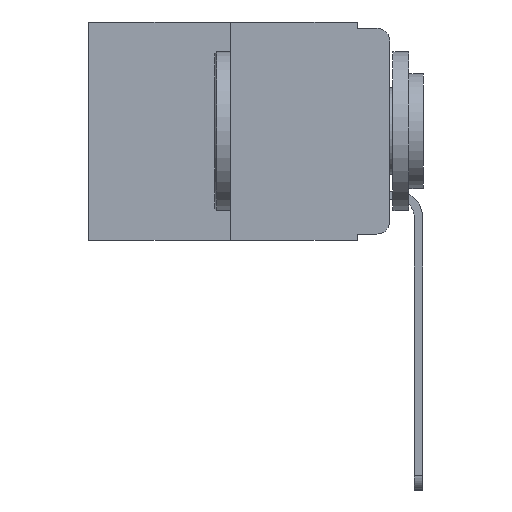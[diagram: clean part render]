
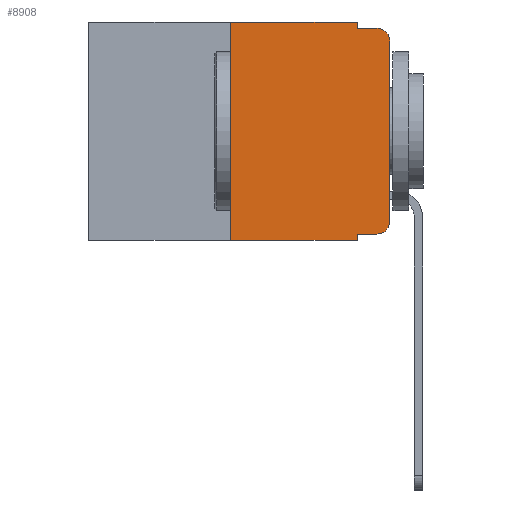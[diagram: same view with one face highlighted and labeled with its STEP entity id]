
A CAD part, left-side view. The second image highlights one B-rep face of the part: STEP entity #8908.
In plain terms, the highlighted planar face has unit normal (-1, 0, 0).
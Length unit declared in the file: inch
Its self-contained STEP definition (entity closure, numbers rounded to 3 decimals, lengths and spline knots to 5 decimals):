
#420 = CARTESIAN_POINT ( 'NONE',  ( 0., 0.473, 0. ) ) ;
#511 = CARTESIAN_POINT ( 'NONE',  ( 0., 0.051, -0.333 ) ) ;
#527 = AXIS2_PLACEMENT_3D ( 'NONE', #420, #4409, #4453 ) ;
#925 = CARTESIAN_POINT ( 'NONE',  ( 0., 0.051, -0.01 ) ) ;
#1046 = VECTOR ( 'NONE', #10687, 39.37008 ) ;
#1094 = DIRECTION ( 'NONE',  ( 0., 0., -1. ) ) ;
#1204 = LINE ( 'NONE', #7359, #10614 ) ;
#1494 = VERTEX_POINT ( 'NONE', #3408 ) ;
#1612 = CARTESIAN_POINT ( 'NONE',  ( 0., 0.02, -0.01 ) ) ;
#1719 = AXIS2_PLACEMENT_3D ( 'NONE', #12759, #5853, #1752 ) ;
#1752 = DIRECTION ( 'NONE',  ( 0., 0., -1. ) ) ;
#1886 = ORIENTED_EDGE ( 'NONE', *, *, #8521, .T. ) ;
#1899 = CARTESIAN_POINT ( 'NONE',  ( 0., 0.02, -0.03 ) ) ;
#1939 = ORIENTED_EDGE ( 'NONE', *, *, #9446, .T. ) ;
#1978 = DIRECTION ( 'NONE',  ( 0., 0., -1. ) ) ;
#2279 = CARTESIAN_POINT ( 'NONE',  ( 0., 0., 0. ) ) ;
#2830 = VERTEX_POINT ( 'NONE', #925 ) ;
#2940 = VERTEX_POINT ( 'NONE', #6816 ) ;
#2972 = EDGE_CURVE ( 'NONE', #7013, #5852, #4363, .T. ) ;
#3397 = EDGE_CURVE ( 'NONE', #2940, #4117, #1204, .T. ) ;
#3408 = CARTESIAN_POINT ( 'NONE',  ( 0., 0.25, -0.343 ) ) ;
#3981 = ORIENTED_EDGE ( 'NONE', *, *, #4809, .F. ) ;
#4117 = VERTEX_POINT ( 'NONE', #8091 ) ;
#4363 = LINE ( 'NONE', #10777, #1046 ) ;
#4409 = DIRECTION ( 'NONE',  ( 1., 0., 0. ) ) ;
#4453 = DIRECTION ( 'NONE',  ( 0., 0., -1. ) ) ;
#4462 = LINE ( 'NONE', #2279, #7758 ) ;
#4608 = VERTEX_POINT ( 'NONE', #1612 ) ;
#4751 = VERTEX_POINT ( 'NONE', #5186 ) ;
#4809 = EDGE_CURVE ( 'NONE', #4117, #2830, #5350, .T. ) ;
#4914 = EDGE_CURVE ( 'NONE', #2830, #4608, #7776, .T. ) ;
#4993 = VECTOR ( 'NONE', #1094, 39.37008 ) ;
#5142 = ORIENTED_EDGE ( 'NONE', *, *, #10206, .F. ) ;
#5186 = CARTESIAN_POINT ( 'NONE',  ( 0., 0., -0.313 ) ) ;
#5350 = LINE ( 'NONE', #7104, #4993 ) ;
#5352 = DIRECTION ( 'NONE',  ( 0., 0., 1. ) ) ;
#5421 = EDGE_LOOP ( 'NONE', ( #1939, #5824, #5986, #3981, #7774, #5142, #8669, #10131, #1886, #11027 ) ) ;
#5438 = LINE ( 'NONE', #511, #6034 ) ;
#5660 = CARTESIAN_POINT ( 'NONE',  ( 0., 0.25, 0. ) ) ;
#5824 = ORIENTED_EDGE ( 'NONE', *, *, #7641, .T. ) ;
#5852 = VERTEX_POINT ( 'NONE', #10627 ) ;
#5853 = DIRECTION ( 'NONE',  ( -1., 0., 0. ) ) ;
#5986 = ORIENTED_EDGE ( 'NONE', *, *, #4914, .F. ) ;
#6007 = VECTOR ( 'NONE', #9472, 39.37008 ) ;
#6034 = VECTOR ( 'NONE', #12544, 39.37008 ) ;
#6197 = FACE_OUTER_BOUND ( 'NONE', #5421, .T. ) ;
#6322 = DIRECTION ( 'NONE',  ( 0., -1., 0. ) ) ;
#6383 = CIRCLE ( 'NONE', #1719, 0.02 ) ;
#6440 = CARTESIAN_POINT ( 'NONE',  ( 0., 0.051, -0.333 ) ) ;
#6643 = AXIS2_PLACEMENT_3D ( 'NONE', #1899, #9906, #1978 ) ;
#6657 = VERTEX_POINT ( 'NONE', #12770 ) ;
#6816 = CARTESIAN_POINT ( 'NONE',  ( 0., 0.25, 0. ) ) ;
#7013 = VERTEX_POINT ( 'NONE', #6440 ) ;
#7095 = VECTOR ( 'NONE', #9711, 39.37008 ) ;
#7104 = CARTESIAN_POINT ( 'NONE',  ( 0., 0.051, 0. ) ) ;
#7246 = DIRECTION ( 'NONE',  ( 0., -1., 0. ) ) ;
#7295 = CARTESIAN_POINT ( 'NONE',  ( 0., 0.051, -0.01 ) ) ;
#7359 = CARTESIAN_POINT ( 'NONE',  ( 0., 0.473, 0. ) ) ;
#7443 = PLANE ( 'NONE',  #527 ) ;
#7641 = EDGE_CURVE ( 'NONE', #6657, #4608, #7931, .T. ) ;
#7661 = CARTESIAN_POINT ( 'NONE',  ( 0., 0.02, -0.333 ) ) ;
#7758 = VECTOR ( 'NONE', #5352, 39.37008 ) ;
#7774 = ORIENTED_EDGE ( 'NONE', *, *, #3397, .F. ) ;
#7776 = LINE ( 'NONE', #7295, #12130 ) ;
#7931 = CIRCLE ( 'NONE', #6643, 0.02 ) ;
#8091 = CARTESIAN_POINT ( 'NONE',  ( 0., 0.051, 0. ) ) ;
#8118 = EDGE_CURVE ( 'NONE', #11606, #4751, #6383, .T. ) ;
#8521 = EDGE_CURVE ( 'NONE', #7013, #11606, #5438, .T. ) ;
#8669 = ORIENTED_EDGE ( 'NONE', *, *, #9628, .T. ) ;
#8820 = LINE ( 'NONE', #5660, #7095 ) ;
#8908 = ADVANCED_FACE ( 'NONE', ( #6197 ), #7443, .F. ) ;
#9446 = EDGE_CURVE ( 'NONE', #4751, #6657, #4462, .T. ) ;
#9472 = DIRECTION ( 'NONE',  ( 0., -1., 0. ) ) ;
#9555 = CARTESIAN_POINT ( 'NONE',  ( 0., 0.473, -0.343 ) ) ;
#9628 = EDGE_CURVE ( 'NONE', #1494, #5852, #11648, .T. ) ;
#9711 = DIRECTION ( 'NONE',  ( 0., 0., 1. ) ) ;
#9906 = DIRECTION ( 'NONE',  ( -1., 0., 0. ) ) ;
#10131 = ORIENTED_EDGE ( 'NONE', *, *, #2972, .F. ) ;
#10206 = EDGE_CURVE ( 'NONE', #1494, #2940, #8820, .T. ) ;
#10614 = VECTOR ( 'NONE', #7246, 39.37008 ) ;
#10627 = CARTESIAN_POINT ( 'NONE',  ( 0., 0.051, -0.343 ) ) ;
#10687 = DIRECTION ( 'NONE',  ( 0., 0., -1. ) ) ;
#10777 = CARTESIAN_POINT ( 'NONE',  ( 0., 0.051, 0. ) ) ;
#11027 = ORIENTED_EDGE ( 'NONE', *, *, #8118, .T. ) ;
#11606 = VERTEX_POINT ( 'NONE', #7661 ) ;
#11648 = LINE ( 'NONE', #9555, #6007 ) ;
#12130 = VECTOR ( 'NONE', #6322, 39.37008 ) ;
#12544 = DIRECTION ( 'NONE',  ( 0., -1., 0. ) ) ;
#12759 = CARTESIAN_POINT ( 'NONE',  ( 0., 0.02, -0.313 ) ) ;
#12770 = CARTESIAN_POINT ( 'NONE',  ( 0., 0., -0.03 ) ) ;
